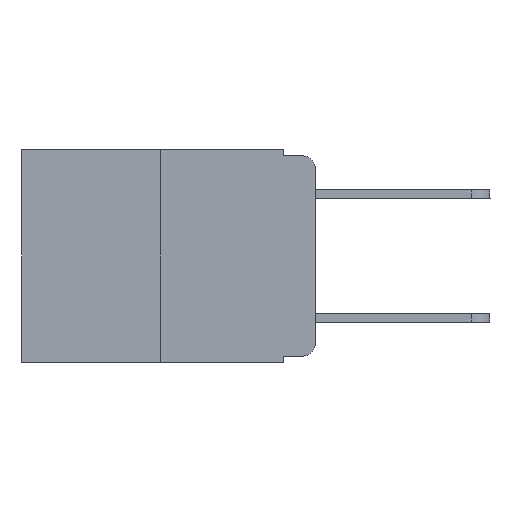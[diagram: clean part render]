
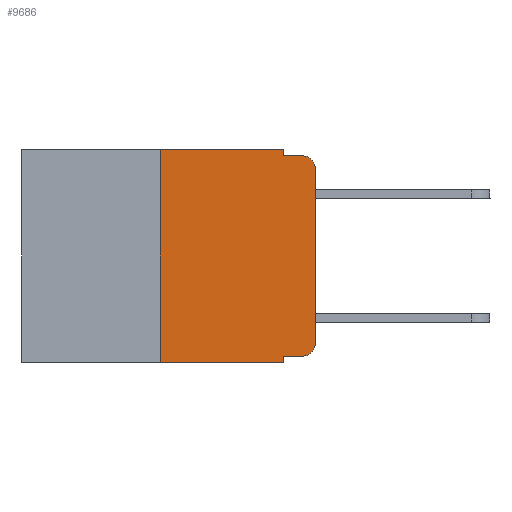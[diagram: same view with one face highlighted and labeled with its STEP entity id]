
A CAD part, left-side view. The second image highlights one B-rep face of the part: STEP entity #9686.
In plain terms, the highlighted planar face has unit normal (-1, 0, 0).
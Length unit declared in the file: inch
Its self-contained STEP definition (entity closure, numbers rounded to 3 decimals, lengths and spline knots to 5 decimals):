
#2 = CARTESIAN_POINT ( 'NONE',  ( 0., 0.02, -0.333 ) ) ;
#227 = CIRCLE ( 'NONE', #8310, 0.02 ) ;
#310 = VECTOR ( 'NONE', #1640, 39.37008 ) ;
#454 = ORIENTED_EDGE ( 'NONE', *, *, #729, .F. ) ;
#463 = CARTESIAN_POINT ( 'NONE',  ( 0., 0.25, 0. ) ) ;
#494 = DIRECTION ( 'NONE',  ( 0., 0., 1. ) ) ;
#705 = CARTESIAN_POINT ( 'NONE',  ( 0., 0.473, -0.343 ) ) ;
#729 = EDGE_CURVE ( 'NONE', #2779, #1281, #1124, .T. ) ;
#915 = ORIENTED_EDGE ( 'NONE', *, *, #2848, .T. ) ;
#1093 = VERTEX_POINT ( 'NONE', #2 ) ;
#1124 = LINE ( 'NONE', #6927, #6649 ) ;
#1197 = DIRECTION ( 'NONE',  ( 0., -1., 0. ) ) ;
#1221 = ORIENTED_EDGE ( 'NONE', *, *, #1878, .T. ) ;
#1281 = VERTEX_POINT ( 'NONE', #4944 ) ;
#1408 = CARTESIAN_POINT ( 'NONE',  ( 0., 0., -0.313 ) ) ;
#1413 = VECTOR ( 'NONE', #4058, 39.37008 ) ;
#1490 = VERTEX_POINT ( 'NONE', #2900 ) ;
#1640 = DIRECTION ( 'NONE',  ( 0., -1., 0. ) ) ;
#1789 = CARTESIAN_POINT ( 'NONE',  ( 0., 0.473, 0. ) ) ;
#1878 = EDGE_CURVE ( 'NONE', #1093, #7131, #227, .T. ) ;
#1893 = ORIENTED_EDGE ( 'NONE', *, *, #7725, .F. ) ;
#2229 = AXIS2_PLACEMENT_3D ( 'NONE', #1789, #5574, #4832 ) ;
#2259 = DIRECTION ( 'NONE',  ( -1., 0., 0. ) ) ;
#2332 = CARTESIAN_POINT ( 'NONE',  ( 0., 0.02, -0.03 ) ) ;
#2343 = FACE_OUTER_BOUND ( 'NONE', #3294, .T. ) ;
#2412 = CARTESIAN_POINT ( 'NONE',  ( 0., 0.051, -0.333 ) ) ;
#2621 = VECTOR ( 'NONE', #9824, 39.37008 ) ;
#2771 = ORIENTED_EDGE ( 'NONE', *, *, #7102, .T. ) ;
#2772 = CARTESIAN_POINT ( 'NONE',  ( 0., 0., 0. ) ) ;
#2779 = VERTEX_POINT ( 'NONE', #2412 ) ;
#2848 = EDGE_CURVE ( 'NONE', #7131, #6396, #9791, .T. ) ;
#2900 = CARTESIAN_POINT ( 'NONE',  ( 0., 0.25, -0.343 ) ) ;
#2920 = CARTESIAN_POINT ( 'NONE',  ( 0., 0.473, 0. ) ) ;
#3294 = EDGE_LOOP ( 'NONE', ( #915, #8679, #5143, #9439, #1893, #9835, #2771, #454, #5380, #1221 ) ) ;
#3387 = LINE ( 'NONE', #9123, #5235 ) ;
#3584 = EDGE_CURVE ( 'NONE', #2779, #1093, #3387, .T. ) ;
#3607 = DIRECTION ( 'NONE',  ( 0., -1., 0. ) ) ;
#3664 = CARTESIAN_POINT ( 'NONE',  ( 0., 0.02, -0.01 ) ) ;
#3712 = CARTESIAN_POINT ( 'NONE',  ( 0., 0.25, 0. ) ) ;
#3851 = LINE ( 'NONE', #463, #2621 ) ;
#3906 = DIRECTION ( 'NONE',  ( -1., 0., 0. ) ) ;
#4058 = DIRECTION ( 'NONE',  ( 0., 0., -1. ) ) ;
#4141 = VECTOR ( 'NONE', #494, 39.37008 ) ;
#4180 = EDGE_CURVE ( 'NONE', #5714, #4308, #5853, .T. ) ;
#4280 = LINE ( 'NONE', #705, #8477 ) ;
#4308 = VERTEX_POINT ( 'NONE', #3664 ) ;
#4485 = EDGE_CURVE ( 'NONE', #5729, #5714, #5085, .T. ) ;
#4772 = VECTOR ( 'NONE', #3607, 39.37008 ) ;
#4832 = DIRECTION ( 'NONE',  ( 0., 0., -1. ) ) ;
#4871 = EDGE_CURVE ( 'NONE', #1490, #9531, #3851, .T. ) ;
#4926 = CARTESIAN_POINT ( 'NONE',  ( 0., 0.051, -0.01 ) ) ;
#4944 = CARTESIAN_POINT ( 'NONE',  ( 0., 0.051, -0.343 ) ) ;
#4945 = PLANE ( 'NONE',  #2229 ) ;
#5085 = LINE ( 'NONE', #5611, #1413 ) ;
#5143 = ORIENTED_EDGE ( 'NONE', *, *, #4180, .F. ) ;
#5235 = VECTOR ( 'NONE', #1197, 39.37008 ) ;
#5283 = EDGE_CURVE ( 'NONE', #6396, #4308, #5452, .T. ) ;
#5380 = ORIENTED_EDGE ( 'NONE', *, *, #3584, .T. ) ;
#5428 = DIRECTION ( 'NONE',  ( 0., 0., -1. ) ) ;
#5452 = CIRCLE ( 'NONE', #7554, 0.02 ) ;
#5574 = DIRECTION ( 'NONE',  ( 1., 0., 0. ) ) ;
#5611 = CARTESIAN_POINT ( 'NONE',  ( 0., 0.051, 0. ) ) ;
#5714 = VERTEX_POINT ( 'NONE', #4926 ) ;
#5729 = VERTEX_POINT ( 'NONE', #8804 ) ;
#5853 = LINE ( 'NONE', #8551, #310 ) ;
#6206 = DIRECTION ( 'NONE',  ( 0., 0., -1. ) ) ;
#6396 = VERTEX_POINT ( 'NONE', #7961 ) ;
#6649 = VECTOR ( 'NONE', #6206, 39.37008 ) ;
#6904 = DIRECTION ( 'NONE',  ( 0., -1., 0. ) ) ;
#6927 = CARTESIAN_POINT ( 'NONE',  ( 0., 0.051, 0. ) ) ;
#7102 = EDGE_CURVE ( 'NONE', #1490, #1281, #4280, .T. ) ;
#7131 = VERTEX_POINT ( 'NONE', #1408 ) ;
#7554 = AXIS2_PLACEMENT_3D ( 'NONE', #2332, #3906, #9388 ) ;
#7725 = EDGE_CURVE ( 'NONE', #9531, #5729, #8705, .T. ) ;
#7803 = CARTESIAN_POINT ( 'NONE',  ( 0., 0.02, -0.313 ) ) ;
#7961 = CARTESIAN_POINT ( 'NONE',  ( 0., 0., -0.03 ) ) ;
#8310 = AXIS2_PLACEMENT_3D ( 'NONE', #7803, #2259, #5428 ) ;
#8477 = VECTOR ( 'NONE', #6904, 39.37008 ) ;
#8551 = CARTESIAN_POINT ( 'NONE',  ( 0., 0.051, -0.01 ) ) ;
#8679 = ORIENTED_EDGE ( 'NONE', *, *, #5283, .T. ) ;
#8705 = LINE ( 'NONE', #2920, #4772 ) ;
#8804 = CARTESIAN_POINT ( 'NONE',  ( 0., 0.051, 0. ) ) ;
#9123 = CARTESIAN_POINT ( 'NONE',  ( 0., 0.051, -0.333 ) ) ;
#9388 = DIRECTION ( 'NONE',  ( 0., 0., -1. ) ) ;
#9439 = ORIENTED_EDGE ( 'NONE', *, *, #4485, .F. ) ;
#9531 = VERTEX_POINT ( 'NONE', #3712 ) ;
#9686 = ADVANCED_FACE ( 'NONE', ( #2343 ), #4945, .F. ) ;
#9791 = LINE ( 'NONE', #2772, #4141 ) ;
#9824 = DIRECTION ( 'NONE',  ( 0., 0., 1. ) ) ;
#9835 = ORIENTED_EDGE ( 'NONE', *, *, #4871, .F. ) ;
